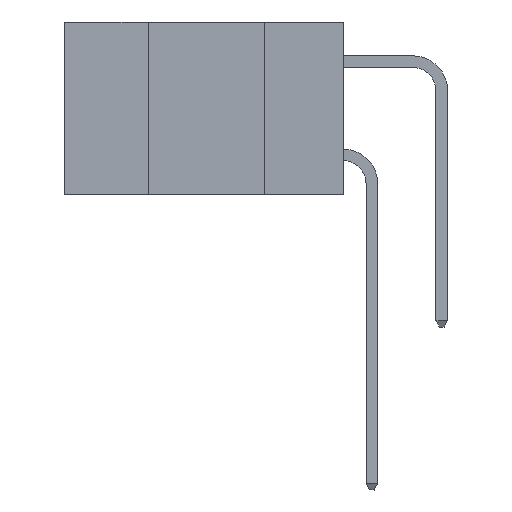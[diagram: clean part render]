
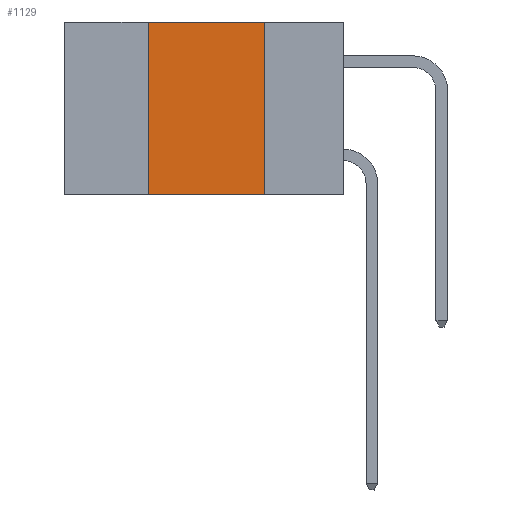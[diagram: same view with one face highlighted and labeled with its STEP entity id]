
A CAD part, left-side view. The second image highlights one B-rep face of the part: STEP entity #1129.
In plain terms, the highlighted planar face has unit normal (-1, 0, 0).
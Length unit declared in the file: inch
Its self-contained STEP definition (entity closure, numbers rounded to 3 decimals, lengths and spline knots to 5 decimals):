
#981 = EDGE_CURVE ( 'NONE', #16093, #9858, #1684, .T. ) ;
#1129 = ADVANCED_FACE ( 'NONE', ( #1360 ), #23744, .F. ) ;
#1360 = FACE_OUTER_BOUND ( 'NONE', #18099, .T. ) ;
#1684 = LINE ( 'NONE', #10709, #20123 ) ;
#2010 = CARTESIAN_POINT ( 'NONE',  ( 0., 0.42, 0. ) ) ;
#2710 = ORIENTED_EDGE ( 'NONE', *, *, #18207, .F. ) ;
#4797 = DIRECTION ( 'NONE',  ( 0., -1., 0. ) ) ;
#5431 = CARTESIAN_POINT ( 'NONE',  ( 0., 0.17, -0.37 ) ) ;
#6361 = CARTESIAN_POINT ( 'NONE',  ( 0., 0.42, -0.37 ) ) ;
#6825 = CARTESIAN_POINT ( 'NONE',  ( 0., 0.6, 0. ) ) ;
#8461 = VERTEX_POINT ( 'NONE', #17797 ) ;
#8517 = CARTESIAN_POINT ( 'NONE',  ( 0., 0.42, 0. ) ) ;
#8877 = DIRECTION ( 'NONE',  ( 1., 0., 0. ) ) ;
#9280 = VECTOR ( 'NONE', #4797, 39.37008 ) ;
#9858 = VERTEX_POINT ( 'NONE', #5431 ) ;
#10466 = VERTEX_POINT ( 'NONE', #2010 ) ;
#10709 = CARTESIAN_POINT ( 'NONE',  ( 0., 0.6, -0.37 ) ) ;
#14229 = DIRECTION ( 'NONE',  ( 0., 0., -1. ) ) ;
#16093 = VERTEX_POINT ( 'NONE', #6361 ) ;
#16291 = CARTESIAN_POINT ( 'NONE',  ( 0., 0.17, 0. ) ) ;
#17243 = CARTESIAN_POINT ( 'NONE',  ( 0., 0.6, 0. ) ) ;
#17797 = CARTESIAN_POINT ( 'NONE',  ( 0., 0.17, 0. ) ) ;
#17821 = EDGE_CURVE ( 'NONE', #16093, #10466, #26088, .T. ) ;
#18029 = AXIS2_PLACEMENT_3D ( 'NONE', #6825, #8877, #23399 ) ;
#18080 = ORIENTED_EDGE ( 'NONE', *, *, #17821, .F. ) ;
#18099 = EDGE_LOOP ( 'NONE', ( #2710, #24980, #18080, #19965 ) ) ;
#18207 = EDGE_CURVE ( 'NONE', #8461, #9858, #24125, .T. ) ;
#18843 = DIRECTION ( 'NONE',  ( 0., 0., 1. ) ) ;
#19128 = DIRECTION ( 'NONE',  ( 0., -1., 0. ) ) ;
#19926 = VECTOR ( 'NONE', #18843, 39.37008 ) ;
#19965 = ORIENTED_EDGE ( 'NONE', *, *, #981, .T. ) ;
#20123 = VECTOR ( 'NONE', #19128, 39.37008 ) ;
#20614 = LINE ( 'NONE', #17243, #9280 ) ;
#23399 = DIRECTION ( 'NONE',  ( 0., 0., -1. ) ) ;
#23512 = EDGE_CURVE ( 'NONE', #10466, #8461, #20614, .T. ) ;
#23744 = PLANE ( 'NONE',  #18029 ) ;
#24125 = LINE ( 'NONE', #16291, #25071 ) ;
#24980 = ORIENTED_EDGE ( 'NONE', *, *, #23512, .F. ) ;
#25071 = VECTOR ( 'NONE', #14229, 39.37008 ) ;
#26088 = LINE ( 'NONE', #8517, #19926 ) ;
